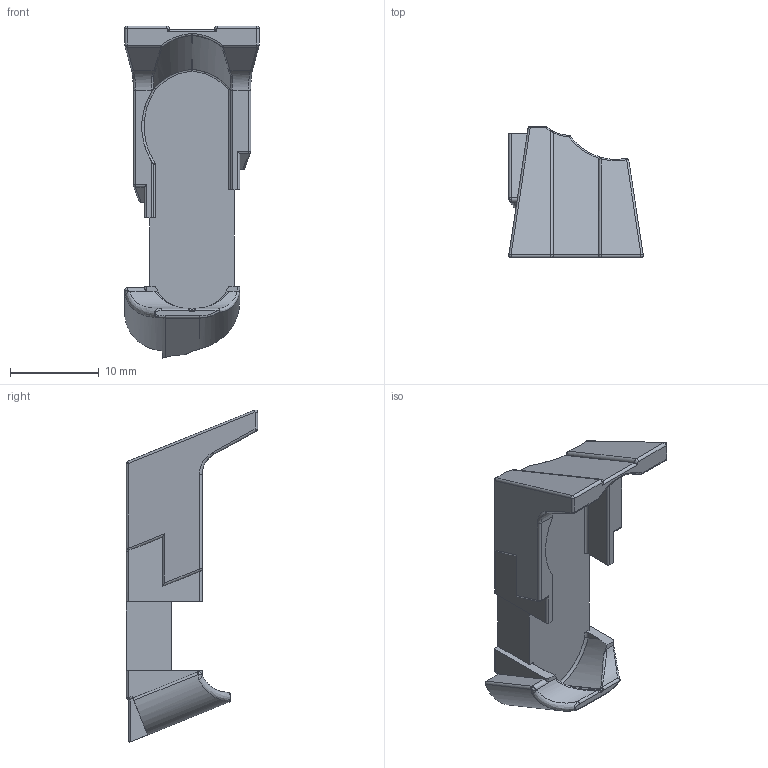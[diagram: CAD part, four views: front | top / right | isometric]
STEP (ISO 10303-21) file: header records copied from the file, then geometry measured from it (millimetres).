
FILE_DESCRIPTION(/* description */ (''),/* implementation_level */ '2;1');
FILE_NAME(/* name */ 'Menendez Mag Follower.stp',/* time_stamp */ '2021-03-20T20:55:12-05:00',/* author */ ('johne'),/* organization */ (''),/* preprocessor_version */ 'ST-DEVELOPER v18',/* originating_system */ 'Autodesk Inventor 2020',/* authorisation */ '');
FILE_SCHEMA (('AUTOMOTIVE_DESIGN { 1 0 10303 214 3 1 1 }'));
Length unit declared in the file: inch
Products named in the file (1): Menendez Mag Follower V1.12
Bounding box: 15.16 x 14.8 x 37.46 mm (x, y, z)
Volume: 1681.7 mm3; surface area: 1754.6 mm2
Topology: 1 solids, 1 shells, 175 faces, 436 edges, 259 vertices
Faces by surface type: cylinder 66, plane 44, bspline 42, sphere 20, torus 3
Entity records: 6477 total; most frequent: CARTESIAN_POINT 2405, ORIENTED_EDGE 864, DIRECTION 837, EDGE_CURVE 432, AXIS2_PLACEMENT_3D 335, VERTEX_POINT 259, FACE_OUTER_BOUND 175, EDGE_LOOP 175
